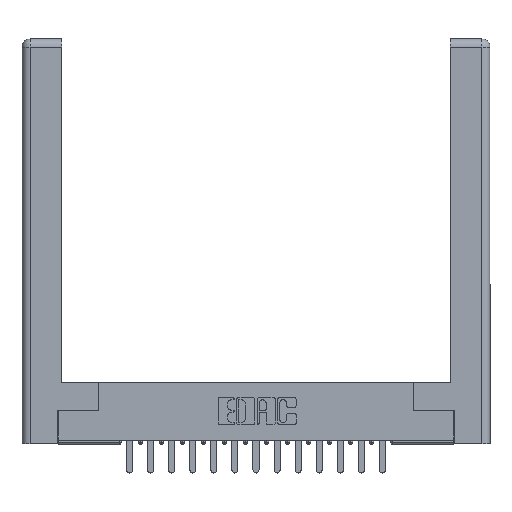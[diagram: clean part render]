
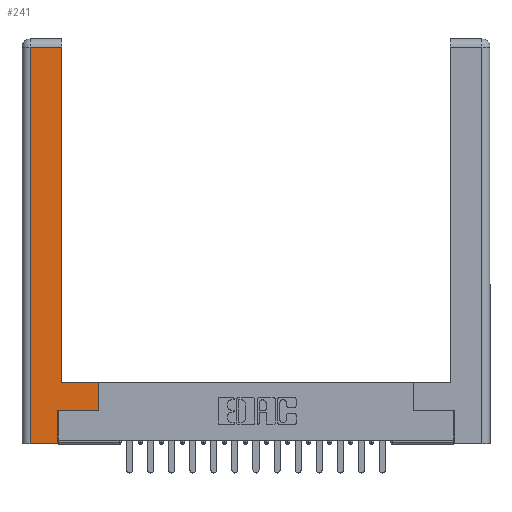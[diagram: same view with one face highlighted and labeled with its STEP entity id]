
A CAD part, top view. The second image highlights one B-rep face of the part: STEP entity #241.
In plain terms, the highlighted planar face has unit normal (0, 0, 1).
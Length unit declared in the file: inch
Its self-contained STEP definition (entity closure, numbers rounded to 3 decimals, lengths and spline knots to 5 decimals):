
#74 = ORIENTED_EDGE ( 'NONE', *, *, #6740, .T. ) ;
#98 = DIRECTION ( 'NONE',  ( -1., 0., 0. ) ) ;
#156 = VECTOR ( 'NONE', #10047, 39.37008 ) ;
#241 = ADVANCED_FACE ( 'NONE', ( #14133 ), #290, .F. ) ;
#264 = CARTESIAN_POINT ( 'NONE',  ( 0.0615, 0., 0. ) ) ;
#290 = PLANE ( 'NONE',  #8578 ) ;
#540 = ORIENTED_EDGE ( 'NONE', *, *, #16307, .T. ) ;
#784 = VERTEX_POINT ( 'NONE', #5916 ) ;
#915 = DIRECTION ( 'NONE',  ( 0., 1., 0. ) ) ;
#938 = CARTESIAN_POINT ( 'NONE',  ( 0.295, 0.45, 0. ) ) ;
#958 = CARTESIAN_POINT ( 'NONE',  ( 0.565, 0.45, 0. ) ) ;
#1408 = VECTOR ( 'NONE', #9914, 39.37008 ) ;
#1482 = CARTESIAN_POINT ( 'NONE',  ( 0.0615, 0., 0. ) ) ;
#2294 = EDGE_CURVE ( 'NONE', #19150, #9946, #19857, .T. ) ;
#2737 = VECTOR ( 'NONE', #915, 39.37008 ) ;
#2954 = LINE ( 'NONE', #7457, #10723 ) ;
#3059 = CARTESIAN_POINT ( 'NONE',  ( 0.265, 0., 0. ) ) ;
#3094 = CARTESIAN_POINT ( 'NONE',  ( 0.565, 0.245, 0. ) ) ;
#3106 = EDGE_CURVE ( 'NONE', #9946, #7183, #4291, .T. ) ;
#3926 = ORIENTED_EDGE ( 'NONE', *, *, #3106, .T. ) ;
#4291 = LINE ( 'NONE', #938, #156 ) ;
#4357 = DIRECTION ( 'NONE',  ( 0., 1., 0. ) ) ;
#4545 = DIRECTION ( 'NONE',  ( 1., 0., 0. ) ) ;
#4630 = VECTOR ( 'NONE', #7675, 39.37008 ) ;
#4916 = CARTESIAN_POINT ( 'NONE',  ( 0.565, 0.245, 0. ) ) ;
#5551 = LINE ( 'NONE', #3059, #6781 ) ;
#5792 = VERTEX_POINT ( 'NONE', #9172 ) ;
#5834 = VERTEX_POINT ( 'NONE', #1482 ) ;
#5878 = VECTOR ( 'NONE', #15578, 39.37008 ) ;
#5916 = CARTESIAN_POINT ( 'NONE',  ( 0.265, 0., 0. ) ) ;
#6255 = LINE ( 'NONE', #264, #16693 ) ;
#6363 = LINE ( 'NONE', #3094, #5878 ) ;
#6390 = ORIENTED_EDGE ( 'NONE', *, *, #16260, .T. ) ;
#6740 = EDGE_CURVE ( 'NONE', #10767, #5834, #6255, .T. ) ;
#6781 = VECTOR ( 'NONE', #4545, 39.37008 ) ;
#6837 = LINE ( 'NONE', #9418, #4630 ) ;
#7183 = VERTEX_POINT ( 'NONE', #7852 ) ;
#7457 = CARTESIAN_POINT ( 'NONE',  ( 0.295, 3., 0. ) ) ;
#7675 = DIRECTION ( 'NONE',  ( -1., 0., 0. ) ) ;
#7852 = CARTESIAN_POINT ( 'NONE',  ( 0.295, 0.45, 0. ) ) ;
#8074 = LINE ( 'NONE', #16128, #2737 ) ;
#8578 = AXIS2_PLACEMENT_3D ( 'NONE', #12823, #12555, #98 ) ;
#9172 = CARTESIAN_POINT ( 'NONE',  ( 0.265, 0.245, 0. ) ) ;
#9418 = CARTESIAN_POINT ( 'NONE',  ( 0.0615, 2.94, 0. ) ) ;
#9551 = EDGE_CURVE ( 'NONE', #5792, #19150, #6363, .T. ) ;
#9595 = ORIENTED_EDGE ( 'NONE', *, *, #2294, .T. ) ;
#9914 = DIRECTION ( 'NONE',  ( 0., 1., 0. ) ) ;
#9946 = VERTEX_POINT ( 'NONE', #958 ) ;
#10047 = DIRECTION ( 'NONE',  ( -1., 0., 0. ) ) ;
#10723 = VECTOR ( 'NONE', #4357, 39.37008 ) ;
#10767 = VERTEX_POINT ( 'NONE', #19088 ) ;
#11262 = CARTESIAN_POINT ( 'NONE',  ( 0.295, 2.94, 0. ) ) ;
#12555 = DIRECTION ( 'NONE',  ( 0., 0., -1. ) ) ;
#12780 = EDGE_CURVE ( 'NONE', #5834, #784, #5551, .T. ) ;
#12823 = CARTESIAN_POINT ( 'NONE',  ( 0., 0., 0. ) ) ;
#13161 = ORIENTED_EDGE ( 'NONE', *, *, #9551, .T. ) ;
#14133 = FACE_OUTER_BOUND ( 'NONE', #19256, .T. ) ;
#15578 = DIRECTION ( 'NONE',  ( 1., 0., 0. ) ) ;
#16128 = CARTESIAN_POINT ( 'NONE',  ( 0.265, 0.245, 0. ) ) ;
#16260 = EDGE_CURVE ( 'NONE', #784, #5792, #8074, .T. ) ;
#16307 = EDGE_CURVE ( 'NONE', #7183, #17163, #2954, .T. ) ;
#16693 = VECTOR ( 'NONE', #17527, 39.37008 ) ;
#17163 = VERTEX_POINT ( 'NONE', #11262 ) ;
#17165 = CARTESIAN_POINT ( 'NONE',  ( 0.565, 0.45, 0. ) ) ;
#17527 = DIRECTION ( 'NONE',  ( 0., -1., 0. ) ) ;
#17560 = EDGE_CURVE ( 'NONE', #17163, #10767, #6837, .T. ) ;
#19088 = CARTESIAN_POINT ( 'NONE',  ( 0.0615, 2.94, 0. ) ) ;
#19150 = VERTEX_POINT ( 'NONE', #4916 ) ;
#19256 = EDGE_LOOP ( 'NONE', ( #540, #19509, #74, #19731, #6390, #13161, #9595, #3926 ) ) ;
#19509 = ORIENTED_EDGE ( 'NONE', *, *, #17560, .T. ) ;
#19731 = ORIENTED_EDGE ( 'NONE', *, *, #12780, .T. ) ;
#19857 = LINE ( 'NONE', #17165, #1408 ) ;
